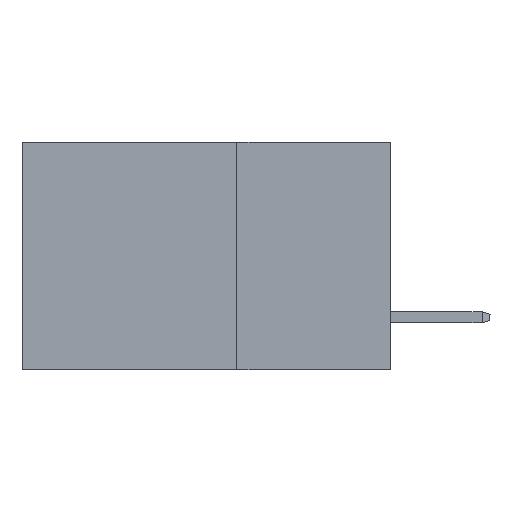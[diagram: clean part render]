
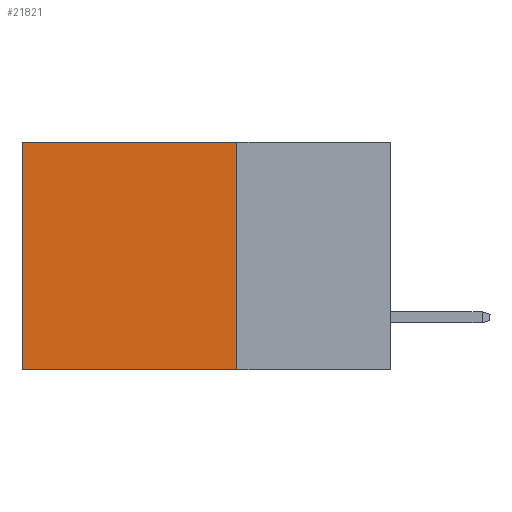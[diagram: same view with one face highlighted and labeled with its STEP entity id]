
A CAD part, left-side view. The second image highlights one B-rep face of the part: STEP entity #21821.
In plain terms, the highlighted planar face has unit normal (-1, 0, 0).
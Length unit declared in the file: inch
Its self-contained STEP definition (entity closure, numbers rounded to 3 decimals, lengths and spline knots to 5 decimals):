
#236 = PLANE ( 'NONE',  #7889 ) ;
#1419 = CARTESIAN_POINT ( 'NONE',  ( 0.2875, 0.25, 0. ) ) ;
#1786 = VERTEX_POINT ( 'NONE', #21694 ) ;
#2027 = DIRECTION ( 'NONE',  ( 0., 0., -1. ) ) ;
#3664 = DIRECTION ( 'NONE',  ( 0., 1., 0. ) ) ;
#3770 = CARTESIAN_POINT ( 'NONE',  ( 0.2875, 0.25, -0.37 ) ) ;
#4056 = VERTEX_POINT ( 'NONE', #1419 ) ;
#4746 = ORIENTED_EDGE ( 'NONE', *, *, #13127, .F. ) ;
#5967 = EDGE_CURVE ( 'NONE', #4056, #20949, #17621, .T. ) ;
#6860 = VECTOR ( 'NONE', #3664, 39.37008 ) ;
#7709 = CARTESIAN_POINT ( 'NONE',  ( 0.2875, 0.25, 0. ) ) ;
#7889 = AXIS2_PLACEMENT_3D ( 'NONE', #22066, #24060, #17907 ) ;
#7947 = CARTESIAN_POINT ( 'NONE',  ( 0.2875, 0.25, -0.37 ) ) ;
#8416 = VERTEX_POINT ( 'NONE', #3770 ) ;
#8493 = ORIENTED_EDGE ( 'NONE', *, *, #9625, .F. ) ;
#9625 = EDGE_CURVE ( 'NONE', #8416, #1786, #21891, .T. ) ;
#9927 = DIRECTION ( 'NONE',  ( 0., 1., 0. ) ) ;
#9953 = LINE ( 'NONE', #21451, #24150 ) ;
#10426 = CARTESIAN_POINT ( 'NONE',  ( 0.2875, 0.6, 0. ) ) ;
#12188 = FACE_OUTER_BOUND ( 'NONE', #21569, .T. ) ;
#13127 = EDGE_CURVE ( 'NONE', #4056, #8416, #16272, .T. ) ;
#13707 = ORIENTED_EDGE ( 'NONE', *, *, #5967, .T. ) ;
#13874 = DIRECTION ( 'NONE',  ( 0., 0., -1. ) ) ;
#16272 = LINE ( 'NONE', #17858, #17835 ) ;
#16622 = VECTOR ( 'NONE', #9927, 39.37008 ) ;
#16993 = EDGE_CURVE ( 'NONE', #20949, #1786, #9953, .T. ) ;
#17621 = LINE ( 'NONE', #7709, #6860 ) ;
#17835 = VECTOR ( 'NONE', #13874, 39.37008 ) ;
#17858 = CARTESIAN_POINT ( 'NONE',  ( 0.2875, 0.25, 0. ) ) ;
#17907 = DIRECTION ( 'NONE',  ( 0., 0., -1. ) ) ;
#20949 = VERTEX_POINT ( 'NONE', #10426 ) ;
#21085 = ORIENTED_EDGE ( 'NONE', *, *, #16993, .T. ) ;
#21451 = CARTESIAN_POINT ( 'NONE',  ( 0.2875, 0.6, 0. ) ) ;
#21569 = EDGE_LOOP ( 'NONE', ( #21085, #8493, #4746, #13707 ) ) ;
#21694 = CARTESIAN_POINT ( 'NONE',  ( 0.2875, 0.6, -0.37 ) ) ;
#21821 = ADVANCED_FACE ( 'NONE', ( #12188 ), #236, .F. ) ;
#21891 = LINE ( 'NONE', #7947, #16622 ) ;
#22066 = CARTESIAN_POINT ( 'NONE',  ( 0.2875, 0.25, 0. ) ) ;
#24060 = DIRECTION ( 'NONE',  ( 1., 0., 0. ) ) ;
#24150 = VECTOR ( 'NONE', #2027, 39.37008 ) ;
